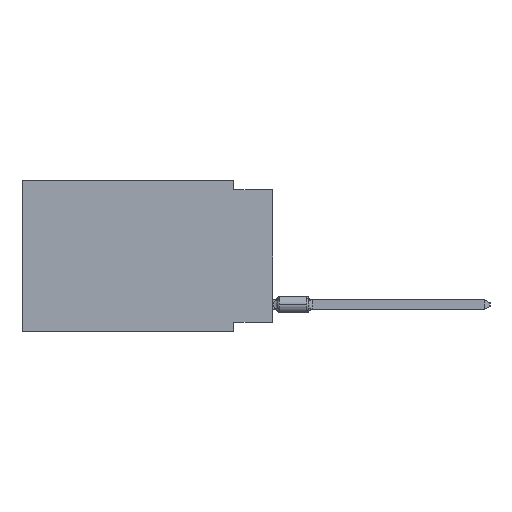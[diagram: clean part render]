
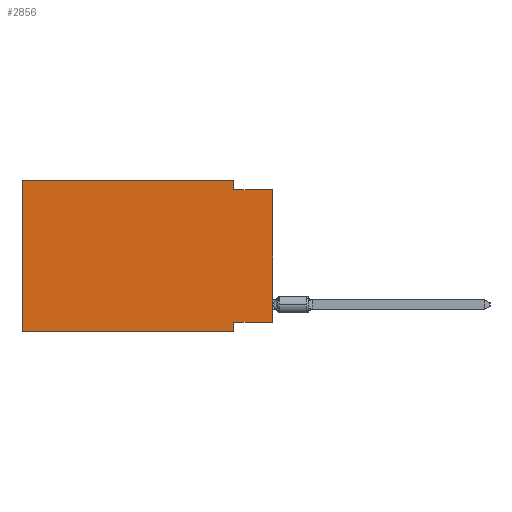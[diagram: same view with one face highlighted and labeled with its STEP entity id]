
A CAD part, left-side view. The second image highlights one B-rep face of the part: STEP entity #2856.
In plain terms, the highlighted planar face has unit normal (-1, 0, 0).
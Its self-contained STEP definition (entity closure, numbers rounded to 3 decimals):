
#141 = VECTOR ( 'NONE', #12964, 1000. ) ;
#171 = ORIENTED_EDGE ( 'NONE', *, *, #21140, .F. ) ;
#581 = VECTOR ( 'NONE', #22445, 1000. ) ;
#991 = EDGE_CURVE ( 'NONE', #7192, #23804, #7566, .T. ) ;
#1405 = CARTESIAN_POINT ( 'NONE',  ( 0., 16.383, 0. ) ) ;
#1894 = LINE ( 'NONE', #27514, #29860 ) ;
#2856 = ADVANCED_FACE ( 'NONE', ( #18733 ), #18555, .F. ) ;
#3324 = CARTESIAN_POINT ( 'NONE',  ( 0., 2.54, -9.906 ) ) ;
#4123 = CARTESIAN_POINT ( 'NONE',  ( 0., 16.383, 0. ) ) ;
#4820 = LINE ( 'NONE', #8038, #581 ) ;
#4892 = VERTEX_POINT ( 'NONE', #32468 ) ;
#4950 = EDGE_CURVE ( 'NONE', #8130, #13424, #6505, .T. ) ;
#5564 = DIRECTION ( 'NONE',  ( 0., 0., -1. ) ) ;
#6505 = LINE ( 'NONE', #18271, #28980 ) ;
#6676 = DIRECTION ( 'NONE',  ( 0., 0., 1. ) ) ;
#6806 = ORIENTED_EDGE ( 'NONE', *, *, #30983, .T. ) ;
#7051 = EDGE_CURVE ( 'NONE', #8130, #4892, #29447, .T. ) ;
#7192 = VERTEX_POINT ( 'NONE', #29995 ) ;
#7566 = LINE ( 'NONE', #10611, #24631 ) ;
#8038 = CARTESIAN_POINT ( 'NONE',  ( 0., 0., -0.635 ) ) ;
#8130 = VERTEX_POINT ( 'NONE', #16801 ) ;
#10205 = DIRECTION ( 'NONE',  ( 1., 0., 0. ) ) ;
#10611 = CARTESIAN_POINT ( 'NONE',  ( 0., 16.383, 0. ) ) ;
#10935 = ORIENTED_EDGE ( 'NONE', *, *, #991, .F. ) ;
#11936 = VECTOR ( 'NONE', #35885, 1000. ) ;
#12964 = DIRECTION ( 'NONE',  ( 0., 0., 1. ) ) ;
#13424 = VERTEX_POINT ( 'NONE', #23367 ) ;
#15236 = VECTOR ( 'NONE', #5564, 1000. ) ;
#15445 = LINE ( 'NONE', #1405, #141 ) ;
#15537 = EDGE_CURVE ( 'NONE', #13424, #36151, #16778, .T. ) ;
#15642 = LINE ( 'NONE', #27190, #11936 ) ;
#16631 = EDGE_CURVE ( 'NONE', #21753, #7192, #15445, .T. ) ;
#16778 = LINE ( 'NONE', #34372, #15236 ) ;
#16801 = CARTESIAN_POINT ( 'NONE',  ( 0., 0., -9.271 ) ) ;
#17031 = VERTEX_POINT ( 'NONE', #33678 ) ;
#18271 = CARTESIAN_POINT ( 'NONE',  ( 0., 0., -9.271 ) ) ;
#18555 = PLANE ( 'NONE',  #25231 ) ;
#18733 = FACE_OUTER_BOUND ( 'NONE', #36733, .T. ) ;
#21105 = DIRECTION ( 'NONE',  ( 0., 1., 0. ) ) ;
#21109 = ORIENTED_EDGE ( 'NONE', *, *, #7051, .T. ) ;
#21140 = EDGE_CURVE ( 'NONE', #17031, #4892, #4820, .T. ) ;
#21421 = CARTESIAN_POINT ( 'NONE',  ( 0., 2.54, 0. ) ) ;
#21556 = DIRECTION ( 'NONE',  ( 0., 0., -1. ) ) ;
#21753 = VERTEX_POINT ( 'NONE', #35614 ) ;
#22445 = DIRECTION ( 'NONE',  ( 0., -1., 0. ) ) ;
#23367 = CARTESIAN_POINT ( 'NONE',  ( 0., 2.54, -9.271 ) ) ;
#23804 = VERTEX_POINT ( 'NONE', #21421 ) ;
#24631 = VECTOR ( 'NONE', #27865, 1000. ) ;
#24894 = EDGE_CURVE ( 'NONE', #23804, #17031, #1894, .T. ) ;
#25231 = AXIS2_PLACEMENT_3D ( 'NONE', #4123, #10205, #21556 ) ;
#27190 = CARTESIAN_POINT ( 'NONE',  ( 0., 16.383, -9.906 ) ) ;
#27254 = ORIENTED_EDGE ( 'NONE', *, *, #24894, .F. ) ;
#27375 = VECTOR ( 'NONE', #6676, 1000. ) ;
#27514 = CARTESIAN_POINT ( 'NONE',  ( 0., 2.54, 0. ) ) ;
#27865 = DIRECTION ( 'NONE',  ( 0., -1., 0. ) ) ;
#28980 = VECTOR ( 'NONE', #21105, 1000. ) ;
#29447 = LINE ( 'NONE', #29624, #27375 ) ;
#29624 = CARTESIAN_POINT ( 'NONE',  ( 0., 0., 0. ) ) ;
#29860 = VECTOR ( 'NONE', #33729, 1000. ) ;
#29995 = CARTESIAN_POINT ( 'NONE',  ( 0., 16.383, 0. ) ) ;
#30983 = EDGE_CURVE ( 'NONE', #21753, #36151, #15642, .T. ) ;
#32468 = CARTESIAN_POINT ( 'NONE',  ( 0., 0., -0.635 ) ) ;
#33571 = ORIENTED_EDGE ( 'NONE', *, *, #4950, .F. ) ;
#33678 = CARTESIAN_POINT ( 'NONE',  ( 0., 2.54, -0.635 ) ) ;
#33729 = DIRECTION ( 'NONE',  ( 0., 0., -1. ) ) ;
#33951 = ORIENTED_EDGE ( 'NONE', *, *, #16631, .F. ) ;
#34180 = ORIENTED_EDGE ( 'NONE', *, *, #15537, .F. ) ;
#34372 = CARTESIAN_POINT ( 'NONE',  ( 0., 2.54, -9.906 ) ) ;
#35614 = CARTESIAN_POINT ( 'NONE',  ( 0., 16.383, -9.906 ) ) ;
#35885 = DIRECTION ( 'NONE',  ( 0., -1., 0. ) ) ;
#36151 = VERTEX_POINT ( 'NONE', #3324 ) ;
#36733 = EDGE_LOOP ( 'NONE', ( #21109, #171, #27254, #10935, #33951, #6806, #34180, #33571 ) ) ;
